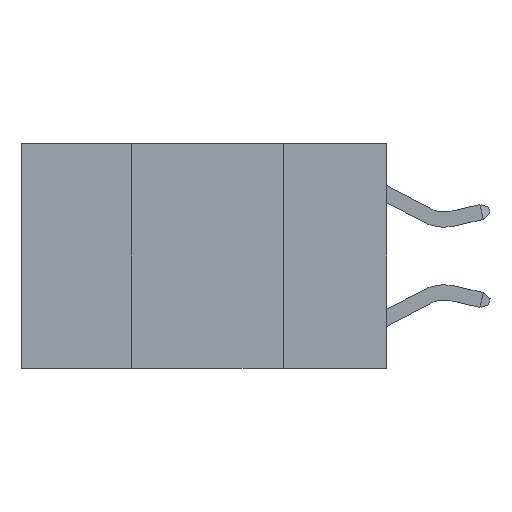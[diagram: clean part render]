
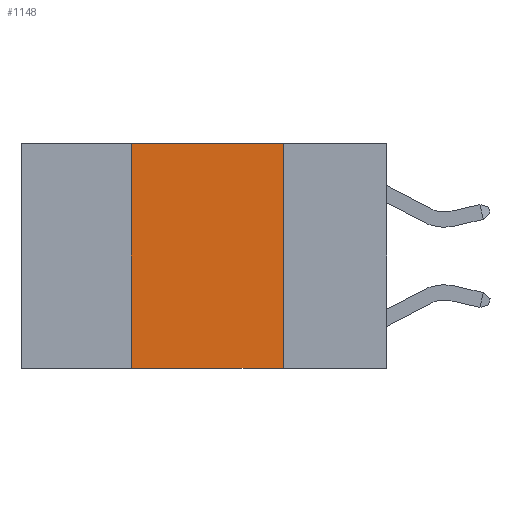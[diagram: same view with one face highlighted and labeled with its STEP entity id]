
A CAD part, left-side view. The second image highlights one B-rep face of the part: STEP entity #1148.
In plain terms, the highlighted planar face has unit normal (-1, 0, 0).
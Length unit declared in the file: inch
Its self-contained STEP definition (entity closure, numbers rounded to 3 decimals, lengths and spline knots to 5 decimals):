
#149 = LINE ( 'NONE', #3455, #4705 ) ;
#247 = CARTESIAN_POINT ( 'NONE',  ( 0., 0.42, 0. ) ) ;
#272 = EDGE_CURVE ( 'NONE', #6536, #7891, #8529, .T. ) ;
#683 = CARTESIAN_POINT ( 'NONE',  ( 0., 0.42, 0. ) ) ;
#789 = CARTESIAN_POINT ( 'NONE',  ( 0., 0.17, 0. ) ) ;
#1148 = ADVANCED_FACE ( 'NONE', ( #5881 ), #4485, .F. ) ;
#1464 = ORIENTED_EDGE ( 'NONE', *, *, #7710, .F. ) ;
#1796 = CARTESIAN_POINT ( 'NONE',  ( 0., 0.6, -0.37 ) ) ;
#1799 = VECTOR ( 'NONE', #2439, 39.37008 ) ;
#2237 = DIRECTION ( 'NONE',  ( 0., 0., -1. ) ) ;
#2439 = DIRECTION ( 'NONE',  ( 0., 0., 1. ) ) ;
#2640 = DIRECTION ( 'NONE',  ( 0., -1., 0. ) ) ;
#2932 = CARTESIAN_POINT ( 'NONE',  ( 0., 0.42, -0.37 ) ) ;
#3000 = CARTESIAN_POINT ( 'NONE',  ( 0., 0.17, 0. ) ) ;
#3455 = CARTESIAN_POINT ( 'NONE',  ( 0., 0.6, 0. ) ) ;
#3668 = ORIENTED_EDGE ( 'NONE', *, *, #9844, .F. ) ;
#4485 = PLANE ( 'NONE',  #9420 ) ;
#4705 = VECTOR ( 'NONE', #5167, 39.37008 ) ;
#5070 = DIRECTION ( 'NONE',  ( 1., 0., 0. ) ) ;
#5167 = DIRECTION ( 'NONE',  ( 0., -1., 0. ) ) ;
#5447 = CARTESIAN_POINT ( 'NONE',  ( 0., 0.17, -0.37 ) ) ;
#5627 = EDGE_CURVE ( 'NONE', #9535, #7891, #7789, .T. ) ;
#5881 = FACE_OUTER_BOUND ( 'NONE', #8020, .T. ) ;
#6260 = LINE ( 'NONE', #683, #1799 ) ;
#6536 = VERTEX_POINT ( 'NONE', #789 ) ;
#7518 = VECTOR ( 'NONE', #2640, 39.37008 ) ;
#7710 = EDGE_CURVE ( 'NONE', #9471, #6536, #149, .T. ) ;
#7789 = LINE ( 'NONE', #1796, #7518 ) ;
#7891 = VERTEX_POINT ( 'NONE', #5447 ) ;
#8020 = EDGE_LOOP ( 'NONE', ( #10075, #1464, #3668, #8159 ) ) ;
#8159 = ORIENTED_EDGE ( 'NONE', *, *, #5627, .T. ) ;
#8529 = LINE ( 'NONE', #3000, #10710 ) ;
#9060 = DIRECTION ( 'NONE',  ( 0., 0., -1. ) ) ;
#9420 = AXIS2_PLACEMENT_3D ( 'NONE', #9528, #5070, #2237 ) ;
#9471 = VERTEX_POINT ( 'NONE', #247 ) ;
#9528 = CARTESIAN_POINT ( 'NONE',  ( 0., 0.6, 0. ) ) ;
#9535 = VERTEX_POINT ( 'NONE', #2932 ) ;
#9844 = EDGE_CURVE ( 'NONE', #9535, #9471, #6260, .T. ) ;
#10075 = ORIENTED_EDGE ( 'NONE', *, *, #272, .F. ) ;
#10710 = VECTOR ( 'NONE', #9060, 39.37008 ) ;
